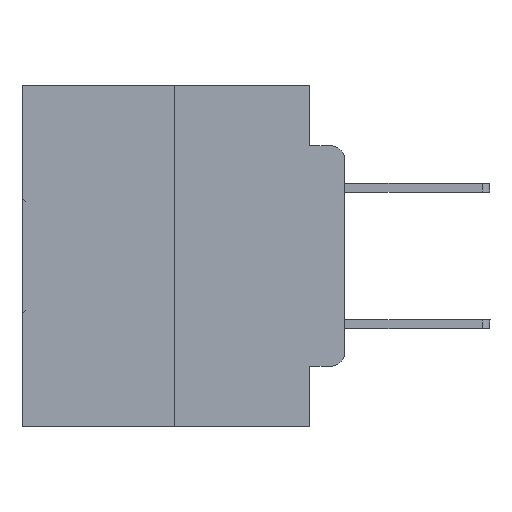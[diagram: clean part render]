
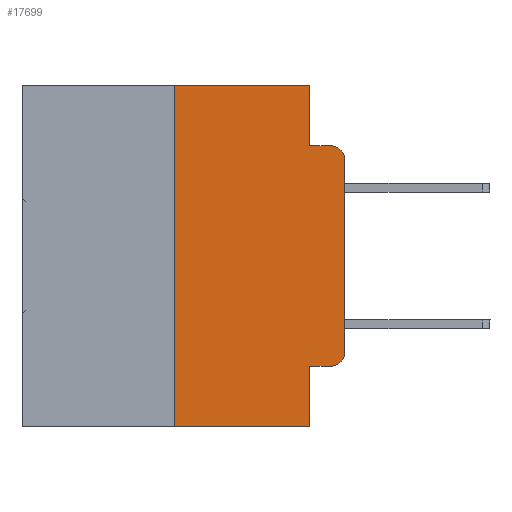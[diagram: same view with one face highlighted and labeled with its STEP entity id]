
A CAD part, left-side view. The second image highlights one B-rep face of the part: STEP entity #17699.
In plain terms, the highlighted planar face has unit normal (-1, 0, 0).
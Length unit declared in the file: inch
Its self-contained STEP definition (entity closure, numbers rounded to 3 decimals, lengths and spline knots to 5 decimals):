
#55 = DIRECTION ( 'NONE',  ( 0., 0., -1. ) ) ;
#281 = CARTESIAN_POINT ( 'NONE',  ( 0., 0.051, 0. ) ) ;
#517 = EDGE_CURVE ( 'NONE', #21955, #8403, #2591, .T. ) ;
#862 = EDGE_CURVE ( 'NONE', #10892, #12764, #24879, .T. ) ;
#1471 = EDGE_CURVE ( 'NONE', #12764, #3640, #22098, .T. ) ;
#2133 = EDGE_CURVE ( 'NONE', #26746, #8403, #18186, .T. ) ;
#2301 = ORIENTED_EDGE ( 'NONE', *, *, #517, .T. ) ;
#2459 = CARTESIAN_POINT ( 'NONE',  ( 0., 0.473, -0.5 ) ) ;
#2591 = CIRCLE ( 'NONE', #10304, 0.02 ) ;
#3640 = VERTEX_POINT ( 'NONE', #14869 ) ;
#4020 = EDGE_CURVE ( 'NONE', #12512, #8655, #29106, .T. ) ;
#4065 = VECTOR ( 'NONE', #25440, 39.37008 ) ;
#4324 = CARTESIAN_POINT ( 'NONE',  ( 0., 0., -0.1085 ) ) ;
#4329 = CARTESIAN_POINT ( 'NONE',  ( 0., 0.25, 0. ) ) ;
#4921 = EDGE_CURVE ( 'NONE', #10892, #16341, #18139, .T. ) ;
#5102 = ORIENTED_EDGE ( 'NONE', *, *, #862, .F. ) ;
#6399 = AXIS2_PLACEMENT_3D ( 'NONE', #31132, #16189, #18667 ) ;
#6632 = CARTESIAN_POINT ( 'NONE',  ( 0., 0.25, 0. ) ) ;
#6653 = DIRECTION ( 'NONE',  ( -1., 0., 0. ) ) ;
#7824 = ORIENTED_EDGE ( 'NONE', *, *, #4020, .T. ) ;
#8379 = DIRECTION ( 'NONE',  ( 0., -1., 0. ) ) ;
#8403 = VERTEX_POINT ( 'NONE', #28362 ) ;
#8655 = VERTEX_POINT ( 'NONE', #11958 ) ;
#8942 = DIRECTION ( 'NONE',  ( 0., -1., 0. ) ) ;
#10037 = FACE_OUTER_BOUND ( 'NONE', #26952, .T. ) ;
#10243 = CARTESIAN_POINT ( 'NONE',  ( 0., 0.02, -0.4115 ) ) ;
#10304 = AXIS2_PLACEMENT_3D ( 'NONE', #16628, #6653, #26853 ) ;
#10892 = VERTEX_POINT ( 'NONE', #12945 ) ;
#11391 = ORIENTED_EDGE ( 'NONE', *, *, #1471, .F. ) ;
#11958 = CARTESIAN_POINT ( 'NONE',  ( 0., 0., -0.3915 ) ) ;
#12121 = CARTESIAN_POINT ( 'NONE',  ( 0., 0.051, -0.5 ) ) ;
#12294 = LINE ( 'NONE', #20405, #4065 ) ;
#12512 = VERTEX_POINT ( 'NONE', #10243 ) ;
#12764 = VERTEX_POINT ( 'NONE', #6632 ) ;
#12945 = CARTESIAN_POINT ( 'NONE',  ( 0., 0.25, -0.5 ) ) ;
#13124 = ORIENTED_EDGE ( 'NONE', *, *, #24438, .F. ) ;
#13546 = VECTOR ( 'NONE', #24429, 39.37008 ) ;
#13897 = VECTOR ( 'NONE', #21537, 39.37008 ) ;
#13905 = VECTOR ( 'NONE', #8379, 39.37008 ) ;
#14408 = EDGE_CURVE ( 'NONE', #19227, #12512, #24928, .T. ) ;
#14856 = CARTESIAN_POINT ( 'NONE',  ( 0., 0.051, 0. ) ) ;
#14869 = CARTESIAN_POINT ( 'NONE',  ( 0., 0.051, 0. ) ) ;
#14887 = ORIENTED_EDGE ( 'NONE', *, *, #23359, .F. ) ;
#15638 = DIRECTION ( 'NONE',  ( 0., 0., -1. ) ) ;
#15640 = CARTESIAN_POINT ( 'NONE',  ( 0., 0.051, -0.0885 ) ) ;
#15919 = LINE ( 'NONE', #281, #20975 ) ;
#16189 = DIRECTION ( 'NONE',  ( -1., 0., 0. ) ) ;
#16341 = VERTEX_POINT ( 'NONE', #12121 ) ;
#16628 = CARTESIAN_POINT ( 'NONE',  ( 0., 0.02, -0.1085 ) ) ;
#16711 = CARTESIAN_POINT ( 'NONE',  ( 0., 0.051, -0.4115 ) ) ;
#17699 = ADVANCED_FACE ( 'NONE', ( #10037 ), #17735, .F. ) ;
#17735 = PLANE ( 'NONE',  #28481 ) ;
#18139 = LINE ( 'NONE', #2459, #22833 ) ;
#18186 = LINE ( 'NONE', #27691, #13905 ) ;
#18579 = ORIENTED_EDGE ( 'NONE', *, *, #4921, .T. ) ;
#18667 = DIRECTION ( 'NONE',  ( 0., 0., -1. ) ) ;
#19227 = VERTEX_POINT ( 'NONE', #16711 ) ;
#20026 = DIRECTION ( 'NONE',  ( 1., 0., 0. ) ) ;
#20405 = CARTESIAN_POINT ( 'NONE',  ( 0., 0., 0. ) ) ;
#20975 = VECTOR ( 'NONE', #15638, 39.37008 ) ;
#21537 = DIRECTION ( 'NONE',  ( 0., -1., 0. ) ) ;
#21955 = VERTEX_POINT ( 'NONE', #4324 ) ;
#22083 = CARTESIAN_POINT ( 'NONE',  ( 0., 0.473, 0. ) ) ;
#22098 = LINE ( 'NONE', #22083, #13897 ) ;
#22363 = ORIENTED_EDGE ( 'NONE', *, *, #14408, .T. ) ;
#22507 = DIRECTION ( 'NONE',  ( 0., -1., 0. ) ) ;
#22561 = DIRECTION ( 'NONE',  ( 0., 0., -1. ) ) ;
#22833 = VECTOR ( 'NONE', #22507, 39.37008 ) ;
#22976 = ORIENTED_EDGE ( 'NONE', *, *, #2133, .F. ) ;
#23359 = EDGE_CURVE ( 'NONE', #19227, #16341, #15919, .T. ) ;
#24429 = DIRECTION ( 'NONE',  ( 0., 0., 1. ) ) ;
#24438 = EDGE_CURVE ( 'NONE', #3640, #26746, #27122, .T. ) ;
#24879 = LINE ( 'NONE', #4329, #13546 ) ;
#24928 = LINE ( 'NONE', #31669, #30422 ) ;
#25440 = DIRECTION ( 'NONE',  ( 0., 0., 1. ) ) ;
#26726 = VECTOR ( 'NONE', #55, 39.37008 ) ;
#26746 = VERTEX_POINT ( 'NONE', #15640 ) ;
#26853 = DIRECTION ( 'NONE',  ( 0., 0., -1. ) ) ;
#26952 = EDGE_LOOP ( 'NONE', ( #30727, #2301, #22976, #13124, #11391, #5102, #18579, #14887, #22363, #7824 ) ) ;
#27122 = LINE ( 'NONE', #14856, #26726 ) ;
#27691 = CARTESIAN_POINT ( 'NONE',  ( 0., 0.051, -0.0885 ) ) ;
#28362 = CARTESIAN_POINT ( 'NONE',  ( 0., 0.02, -0.0885 ) ) ;
#28481 = AXIS2_PLACEMENT_3D ( 'NONE', #29959, #20026, #22561 ) ;
#28503 = EDGE_CURVE ( 'NONE', #8655, #21955, #12294, .T. ) ;
#29106 = CIRCLE ( 'NONE', #6399, 0.02 ) ;
#29959 = CARTESIAN_POINT ( 'NONE',  ( 0., 0.473, 0. ) ) ;
#30422 = VECTOR ( 'NONE', #8942, 39.37008 ) ;
#30727 = ORIENTED_EDGE ( 'NONE', *, *, #28503, .T. ) ;
#31132 = CARTESIAN_POINT ( 'NONE',  ( 0., 0.02, -0.3915 ) ) ;
#31669 = CARTESIAN_POINT ( 'NONE',  ( 0., 0.051, -0.4115 ) ) ;
